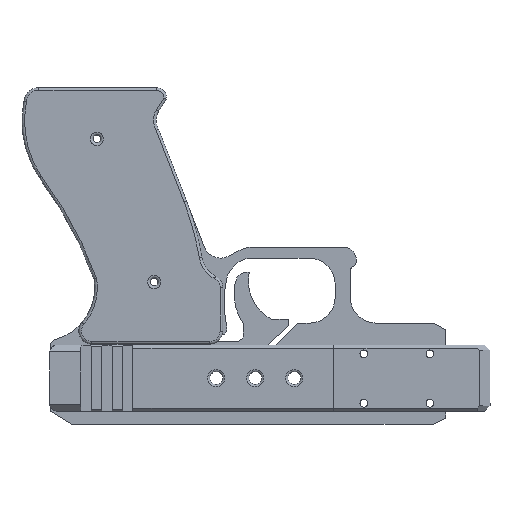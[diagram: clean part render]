
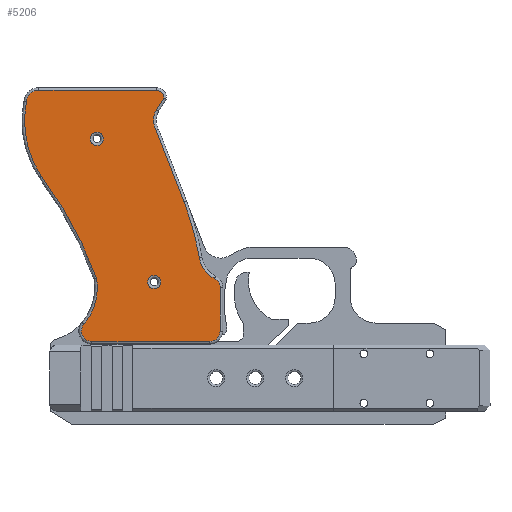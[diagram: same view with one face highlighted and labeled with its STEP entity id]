
A CAD part, front view. The second image highlights one B-rep face of the part: STEP entity #5206.
In plain terms, the highlighted face is planar.
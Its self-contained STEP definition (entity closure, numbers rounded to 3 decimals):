
#173=FACE_BOUND('',#895,.T.);
#174=FACE_BOUND('',#896,.T.);
#318=PLANE('',#5764);
#565=FACE_OUTER_BOUND('',#894,.T.);
#894=EDGE_LOOP('',(#4693,#4694,#4695,#4696,#4697,#4698,#4699,#4700,#4701,
#4702,#4703,#4704,#4705,#4706,#4707,#4708));
#895=EDGE_LOOP('',(#4709));
#896=EDGE_LOOP('',(#4710));
#1396=LINE('',#8861,#1890);
#1397=LINE('',#8865,#1891);
#1398=LINE('',#8873,#1892);
#1399=LINE('',#8877,#1893);
#1400=LINE('',#8881,#1894);
#1890=VECTOR('',#7194,10.);
#1891=VECTOR('',#7197,10.);
#1892=VECTOR('',#7204,10.);
#1893=VECTOR('',#7207,10.);
#1894=VECTOR('',#7210,10.);
#2104=CIRCLE('',#5761,2.5);
#2107=CIRCLE('',#5765,21.661);
#2108=CIRCLE('',#5766,4.);
#2109=CIRCLE('',#5767,4.);
#2110=CIRCLE('',#5768,4.);
#2111=CIRCLE('',#5769,11.);
#2112=CIRCLE('',#5770,107.);
#2113=CIRCLE('',#5771,7.989);
#2114=CIRCLE('',#5772,2.688);
#2115=CIRCLE('',#5773,4.634);
#2116=CIRCLE('',#5774,38.025);
#2117=CIRCLE('',#5775,154.545);
#2118=CIRCLE('',#5776,2.5);
#2581=VERTEX_POINT('',#8849);
#2583=VERTEX_POINT('',#8855);
#2584=VERTEX_POINT('',#8856);
#2585=VERTEX_POINT('',#8858);
#2586=VERTEX_POINT('',#8860);
#2587=VERTEX_POINT('',#8862);
#2588=VERTEX_POINT('',#8864);
#2589=VERTEX_POINT('',#8866);
#2590=VERTEX_POINT('',#8868);
#2591=VERTEX_POINT('',#8870);
#2592=VERTEX_POINT('',#8872);
#2593=VERTEX_POINT('',#8874);
#2594=VERTEX_POINT('',#8876);
#2595=VERTEX_POINT('',#8878);
#2596=VERTEX_POINT('',#8880);
#2597=VERTEX_POINT('',#8882);
#2598=VERTEX_POINT('',#8884);
#2599=VERTEX_POINT('',#8887);
#3290=EDGE_CURVE('',#2581,#2581,#2104,.T.);
#3293=EDGE_CURVE('',#2583,#2584,#2107,.T.);
#3294=EDGE_CURVE('',#2585,#2583,#2108,.T.);
#3295=EDGE_CURVE('',#2586,#2585,#1396,.T.);
#3296=EDGE_CURVE('',#2587,#2586,#2109,.T.);
#3297=EDGE_CURVE('',#2588,#2587,#1397,.T.);
#3298=EDGE_CURVE('',#2589,#2588,#2110,.T.);
#3299=EDGE_CURVE('',#2590,#2589,#2111,.T.);
#3300=EDGE_CURVE('',#2591,#2590,#2112,.T.);
#3301=EDGE_CURVE('',#2592,#2591,#1398,.T.);
#3302=EDGE_CURVE('',#2593,#2592,#2113,.T.);
#3303=EDGE_CURVE('',#2594,#2593,#1399,.T.);
#3304=EDGE_CURVE('',#2595,#2594,#2114,.T.);
#3305=EDGE_CURVE('',#2596,#2595,#1400,.T.);
#3306=EDGE_CURVE('',#2597,#2596,#2115,.T.);
#3307=EDGE_CURVE('',#2598,#2597,#2116,.T.);
#3308=EDGE_CURVE('',#2584,#2598,#2117,.T.);
#3309=EDGE_CURVE('',#2599,#2599,#2118,.T.);
#4693=ORIENTED_EDGE('',*,*,#3293,.F.);
#4694=ORIENTED_EDGE('',*,*,#3294,.F.);
#4695=ORIENTED_EDGE('',*,*,#3295,.F.);
#4696=ORIENTED_EDGE('',*,*,#3296,.F.);
#4697=ORIENTED_EDGE('',*,*,#3297,.F.);
#4698=ORIENTED_EDGE('',*,*,#3298,.F.);
#4699=ORIENTED_EDGE('',*,*,#3299,.F.);
#4700=ORIENTED_EDGE('',*,*,#3300,.F.);
#4701=ORIENTED_EDGE('',*,*,#3301,.F.);
#4702=ORIENTED_EDGE('',*,*,#3302,.F.);
#4703=ORIENTED_EDGE('',*,*,#3303,.F.);
#4704=ORIENTED_EDGE('',*,*,#3304,.F.);
#4705=ORIENTED_EDGE('',*,*,#3305,.F.);
#4706=ORIENTED_EDGE('',*,*,#3306,.F.);
#4707=ORIENTED_EDGE('',*,*,#3307,.F.);
#4708=ORIENTED_EDGE('',*,*,#3308,.F.);
#4709=ORIENTED_EDGE('',*,*,#3309,.F.);
#4710=ORIENTED_EDGE('',*,*,#3290,.F.);
#5206=ADVANCED_FACE('',(#565,#173,#174),#318,.T.);
#5761=AXIS2_PLACEMENT_3D('',#8850,#7182,#7183);
#5764=AXIS2_PLACEMENT_3D('',#8854,#7188,#7189);
#5765=AXIS2_PLACEMENT_3D('',#8857,#7190,#7191);
#5766=AXIS2_PLACEMENT_3D('',#8859,#7192,#7193);
#5767=AXIS2_PLACEMENT_3D('',#8863,#7195,#7196);
#5768=AXIS2_PLACEMENT_3D('',#8867,#7198,#7199);
#5769=AXIS2_PLACEMENT_3D('',#8869,#7200,#7201);
#5770=AXIS2_PLACEMENT_3D('',#8871,#7202,#7203);
#5771=AXIS2_PLACEMENT_3D('',#8875,#7205,#7206);
#5772=AXIS2_PLACEMENT_3D('',#8879,#7208,#7209);
#5773=AXIS2_PLACEMENT_3D('',#8883,#7211,#7212);
#5774=AXIS2_PLACEMENT_3D('',#8885,#7213,#7214);
#5775=AXIS2_PLACEMENT_3D('',#8886,#7215,#7216);
#5776=AXIS2_PLACEMENT_3D('',#8888,#7217,#7218);
#7182=DIRECTION('center_axis',(0.,0.,-1.));
#7183=DIRECTION('ref_axis',(1.,0.,0.));
#7188=DIRECTION('center_axis',(0.,0.,-1.));
#7189=DIRECTION('ref_axis',(-1.,0.,0.));
#7190=DIRECTION('center_axis',(0.,0.,-1.));
#7191=DIRECTION('ref_axis',(0.962,0.272,0.));
#7192=DIRECTION('center_axis',(0.,0.,1.));
#7193=DIRECTION('ref_axis',(-0.908,0.418,0.));
#7194=DIRECTION('',(-1.,0.,0.));
#7195=DIRECTION('center_axis',(0.,0.,1.));
#7196=DIRECTION('ref_axis',(0.707,0.707,0.));
#7197=DIRECTION('',(0.,1.,0.));
#7198=DIRECTION('center_axis',(0.,0.,1.));
#7199=DIRECTION('ref_axis',(0.853,-0.522,0.));
#7200=DIRECTION('center_axis',(0.,0.,-1.));
#7201=DIRECTION('ref_axis',(-0.808,0.59,0.));
#7202=DIRECTION('center_axis',(0.,0.,1.));
#7203=DIRECTION('ref_axis',(0.964,-0.264,0.));
#7204=DIRECTION('',(0.363,0.932,0.));
#7205=DIRECTION('center_axis',(0.,0.,-1.));
#7206=DIRECTION('ref_axis',(-1.,-0.016,0.));
#7207=DIRECTION('',(-0.527,0.85,0.));
#7208=DIRECTION('center_axis',(0.,0.,1.));
#7209=DIRECTION('ref_axis',(0.749,-0.662,0.));
#7210=DIRECTION('',(1.,0.,0.));
#7211=DIRECTION('center_axis',(0.,0.,1.));
#7212=DIRECTION('ref_axis',(-0.667,-0.745,0.));
#7213=DIRECTION('center_axis',(0.,0.,1.));
#7214=DIRECTION('ref_axis',(-0.98,0.198,0.));
#7215=DIRECTION('center_axis',(0.,0.,-1.));
#7216=DIRECTION('ref_axis',(0.88,-0.476,0.));
#7217=DIRECTION('center_axis',(0.,0.,-1.));
#7218=DIRECTION('ref_axis',(1.,0.,0.));
#8849=CARTESIAN_POINT('',(19.74,19.64,-2.));
#8850=CARTESIAN_POINT('Origin',(22.24,19.64,-2.));
#8854=CARTESIAN_POINT('Origin',(0.787,76.82,-2.));
#8855=CARTESIAN_POINT('',(17.248,90.9,-2.));
#8856=CARTESIAN_POINT('',(22.168,73.348,-2.));
#8857=CARTESIAN_POINT('Origin',(0.787,76.82,-2.));
#8858=CARTESIAN_POINT('',(20.287,97.5,-2.));
#8859=CARTESIAN_POINT('Origin',(20.287,93.5,-2.));
#8860=CARTESIAN_POINT('',(65.609,97.5,-2.));
#8861=CARTESIAN_POINT('',(32.198,97.5,-2.));
#8862=CARTESIAN_POINT('',(69.609,93.5,-2.));
#8863=CARTESIAN_POINT('Origin',(65.609,93.5,-2.));
#8864=CARTESIAN_POINT('',(69.609,76.873,-2.));
#8865=CARTESIAN_POINT('',(69.609,38.41,-2.));
#8866=CARTESIAN_POINT('',(67.432,73.312,-2.));
#8867=CARTESIAN_POINT('Origin',(65.609,76.873,-2.));
#8868=CARTESIAN_POINT('',(61.591,65.31,-2.));
#8869=CARTESIAN_POINT('Origin',(72.445,63.521,-2.));
#8870=CARTESIAN_POINT('',(55.701,43.828,-2.));
#8871=CARTESIAN_POINT('Origin',(-43.985,82.709,-2.));
#8872=CARTESIAN_POINT('',(45.012,16.423,-2.));
#8873=CARTESIAN_POINT('',(52.303,35.116,-2.));
#8874=CARTESIAN_POINT('',(45.182,8.418,-2.));
#8875=CARTESIAN_POINT('Origin',(52.009,12.567,-2.));
#8876=CARTESIAN_POINT('',(47.931,3.985,-2.));
#8877=CARTESIAN_POINT('',(25.125,40.756,-2.));
#8878=CARTESIAN_POINT('',(45.086,1.,-2.));
#8879=CARTESIAN_POINT('Origin',(45.26,3.683,-2.));
#8880=CARTESIAN_POINT('',(-0.019,1.,-2.));
#8881=CARTESIAN_POINT('',(0.394,1.,-2.));
#8882=CARTESIAN_POINT('',(-4.825,5.342,-2.));
#8883=CARTESIAN_POINT('Origin',(-0.2,5.631,-2.));
#8884=CARTESIAN_POINT('',(0.938,34.048,-2.));
#8885=CARTESIAN_POINT('Origin',(32.463,12.787,-2.));
#8886=CARTESIAN_POINT('Origin',(-122.993,126.381,-2.));
#8887=CARTESIAN_POINT('',(46.74,74.64,-2.));
#8888=CARTESIAN_POINT('Origin',(44.24,74.64,-2.));
